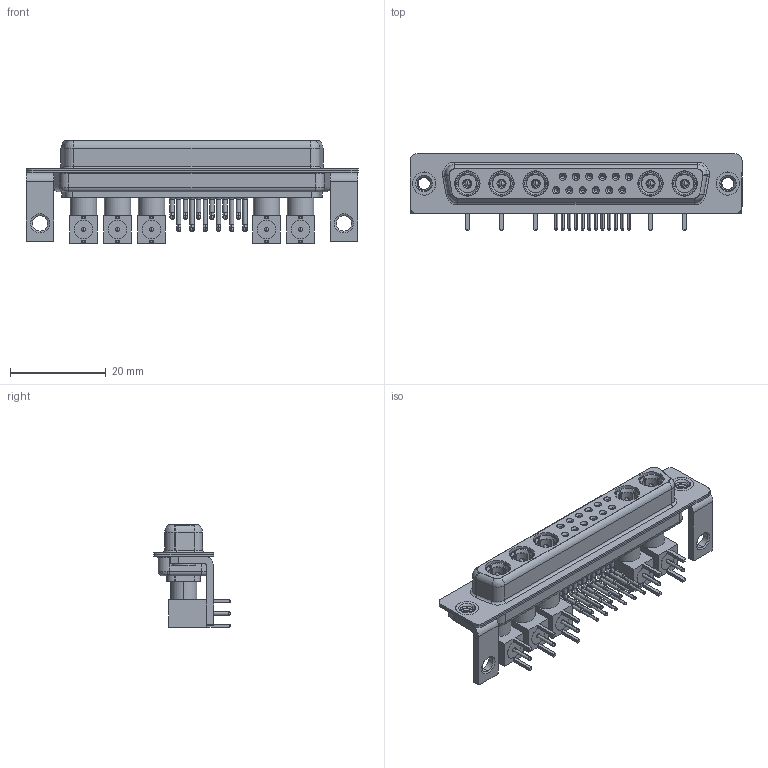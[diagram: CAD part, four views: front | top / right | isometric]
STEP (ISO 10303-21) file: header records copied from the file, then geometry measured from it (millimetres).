
FILE_DESCRIPTION (( 'STEP AP203' ), '1' );
FILE_NAME ('630-17W5640-7TC.STEP', '2022-06-07T00:03:21', ( '' ), ( '' ), 'SwSTEP 2.0', 'SolidWorks 2020', '' );
FILE_SCHEMA (( 'CONFIG_CONTROL_DESIGN' ));
Length unit declared in the file: millimetre
Products named in the file (19): Insulator Pin_Straight PC Tail; 630Combo Contact Row 2; 630Combo Shell Front_37 Contacts; 630Combo Housing_17W5; Co-Ax Plug Assy_RA; Locking Collar; Pin_RA; 630Combo Stabilizer Bracket; 630-17W5640-7TC; Co-Ax Plug_RA PC Tail; 630Combo Threaded Rivet_B; 630Combo Contact Row 1; 630Combo Shell Rear_37 Contacts; Insulator RA Pin; RA Back Shell
Assembly tree (54 placements, depth 3):
  630-17W5640-7TC
    630Combo Housing_17W5
    630Combo Shell Front_37 Contacts
    630Combo Shell Rear_37 Contacts
    630Combo Threaded Rivet_B  x2
    630Combo Stabilizer Bracket  x2
    Co-Ax Plug Assy_RA
      Co-Ax Plug_RA PC Tail
      Insulator Pin_Straight PC Tail
      Pin_RA
      Locking Collar
      RA Back Shell
      Insulator RA Pin
    Co-Ax Plug Assy_RA
      Co-Ax Plug_RA PC Tail
      Insulator Pin_Straight PC Tail
      Pin_RA
      Locking Collar
      RA Back Shell
      Insulator RA Pin
    Co-Ax Plug Assy_RA
      Co-Ax Plug_RA PC Tail
      Insulator Pin_Straight PC Tail
      Pin_RA
      Locking Collar
      RA Back Shell
      Insulator RA Pin
    Co-Ax Plug Assy_RA
      Co-Ax Plug_RA PC Tail
      Insulator Pin_Straight PC Tail
      Pin_RA
      Locking Collar
      RA Back Shell
      Insulator RA Pin
    Co-Ax Plug Assy_RA
      Co-Ax Plug_RA PC Tail
      Insulator Pin_Straight PC Tail
      Pin_RA
      Locking Collar
      RA Back Shell
      Insulator RA Pin
    630Combo Contact Row 1  x6
    630Combo Contact Row 2  x6
Bounding box: 69.4 x 16 x 21.41 mm (x, y, z)
Volume: 6765.2 mm3; surface area: 16079.6 mm2
Topology: 49 solids, 49 shells, 1793 faces, 4410 edges, 2768 vertices
Faces by surface type: cylinder 756, plane 602, cone 269, torus 87, bspline 59, sphere 20
Entity records: 25117 total; most frequent: CARTESIAN_POINT 5434, DIRECTION 3835, ORIENTED_EDGE 3266, EDGE_CURVE 1633, AXIS2_PLACEMENT_3D 1574, VERTEX_POINT 1039, CIRCLE 835, EDGE_LOOP 818
